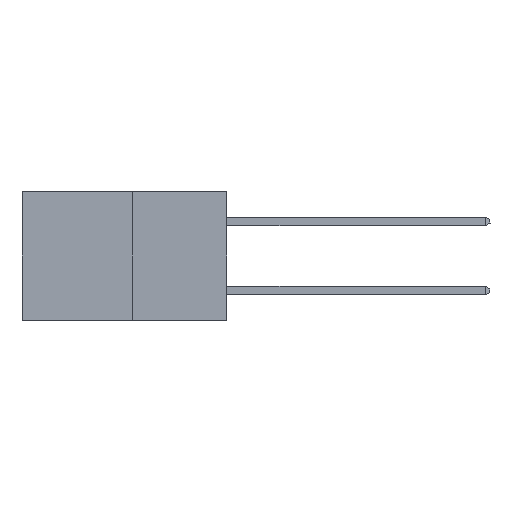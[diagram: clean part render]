
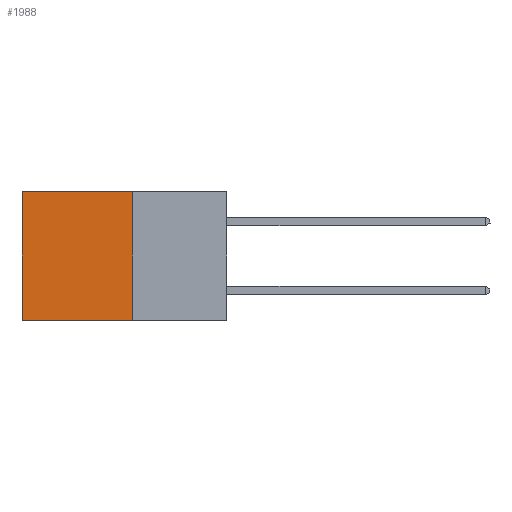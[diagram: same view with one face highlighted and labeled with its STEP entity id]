
A CAD part, left-side view. The second image highlights one B-rep face of the part: STEP entity #1988.
In plain terms, the highlighted planar face has unit normal (-1, 0, 0).
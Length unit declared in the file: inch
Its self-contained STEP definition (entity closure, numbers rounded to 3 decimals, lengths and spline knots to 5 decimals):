
#252 = VERTEX_POINT ( 'NONE', #7718 ) ;
#262 = EDGE_CURVE ( 'NONE', #8495, #4650, #9378, .T. ) ;
#532 = VERTEX_POINT ( 'NONE', #5004 ) ;
#809 = VECTOR ( 'NONE', #2609, 39.37008 ) ;
#1189 = EDGE_CURVE ( 'NONE', #532, #252, #6632, .T. ) ;
#1988 = ADVANCED_FACE ( 'NONE', ( #2445 ), #4981, .F. ) ;
#2241 = LINE ( 'NONE', #8226, #10225 ) ;
#2445 = FACE_OUTER_BOUND ( 'NONE', #9375, .T. ) ;
#2609 = DIRECTION ( 'NONE',  ( 0., 0., -1. ) ) ;
#2811 = CARTESIAN_POINT ( 'NONE',  ( 0.277, 0.59, -0.37 ) ) ;
#3178 = EDGE_CURVE ( 'NONE', #4650, #252, #10043, .T. ) ;
#3203 = CARTESIAN_POINT ( 'NONE',  ( 0.277, 0.27, -0.37 ) ) ;
#3617 = ORIENTED_EDGE ( 'NONE', *, *, #1189, .T. ) ;
#3823 = ORIENTED_EDGE ( 'NONE', *, *, #3178, .F. ) ;
#4025 = AXIS2_PLACEMENT_3D ( 'NONE', #9840, #9565, #10114 ) ;
#4178 = ORIENTED_EDGE ( 'NONE', *, *, #262, .F. ) ;
#4209 = ORIENTED_EDGE ( 'NONE', *, *, #10173, .T. ) ;
#4322 = CARTESIAN_POINT ( 'NONE',  ( 0.277, 0.27, 0. ) ) ;
#4482 = VECTOR ( 'NONE', #6960, 39.37008 ) ;
#4650 = VERTEX_POINT ( 'NONE', #3203 ) ;
#4981 = PLANE ( 'NONE',  #4025 ) ;
#5004 = CARTESIAN_POINT ( 'NONE',  ( 0.277, 0.59, 0. ) ) ;
#6006 = VECTOR ( 'NONE', #6227, 39.37008 ) ;
#6227 = DIRECTION ( 'NONE',  ( 0., 1., 0. ) ) ;
#6511 = CARTESIAN_POINT ( 'NONE',  ( 0.277, 0.27, -0.37 ) ) ;
#6632 = LINE ( 'NONE', #2811, #4482 ) ;
#6819 = DIRECTION ( 'NONE',  ( 0., 1., 0. ) ) ;
#6960 = DIRECTION ( 'NONE',  ( 0., 0., -1. ) ) ;
#7718 = CARTESIAN_POINT ( 'NONE',  ( 0.277, 0.59, -0.37 ) ) ;
#8226 = CARTESIAN_POINT ( 'NONE',  ( 0.277, 0.27, 0. ) ) ;
#8495 = VERTEX_POINT ( 'NONE', #4322 ) ;
#9375 = EDGE_LOOP ( 'NONE', ( #3617, #3823, #4178, #4209 ) ) ;
#9378 = LINE ( 'NONE', #6511, #809 ) ;
#9565 = DIRECTION ( 'NONE',  ( 1., 0., 0. ) ) ;
#9840 = CARTESIAN_POINT ( 'NONE',  ( 0.277, 0.27, -0.37 ) ) ;
#9904 = CARTESIAN_POINT ( 'NONE',  ( 0.277, 0.27, -0.37 ) ) ;
#10043 = LINE ( 'NONE', #9904, #6006 ) ;
#10114 = DIRECTION ( 'NONE',  ( 0., 0., -1. ) ) ;
#10173 = EDGE_CURVE ( 'NONE', #8495, #532, #2241, .T. ) ;
#10225 = VECTOR ( 'NONE', #6819, 39.37008 ) ;
